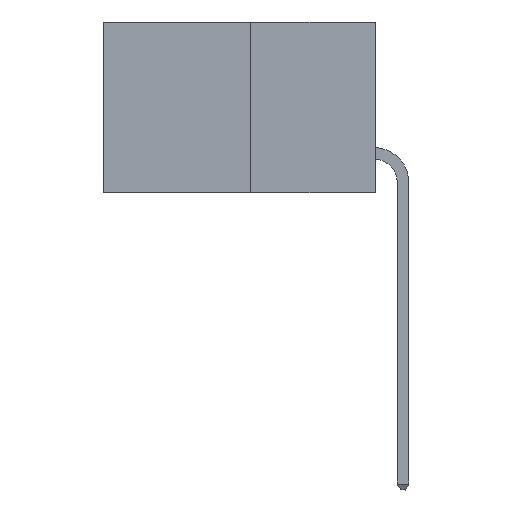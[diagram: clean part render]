
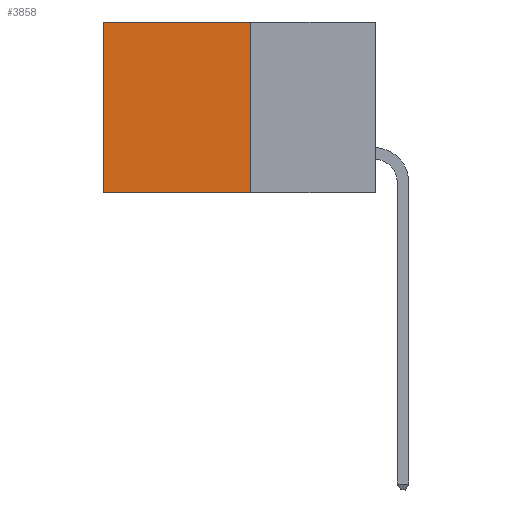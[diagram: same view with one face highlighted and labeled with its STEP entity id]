
A CAD part, left-side view. The second image highlights one B-rep face of the part: STEP entity #3858.
In plain terms, the highlighted planar face has unit normal (-1, 0, 0).
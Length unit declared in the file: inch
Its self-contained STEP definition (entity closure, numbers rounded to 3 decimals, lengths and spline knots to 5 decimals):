
#7 = DIRECTION ( 'NONE',  ( 1., 0., 0. ) ) ;
#21 = CARTESIAN_POINT ( 'NONE',  ( 0.277, 0.59, 0. ) ) ;
#32 = DIRECTION ( 'NONE',  ( 0., 0., -1. ) ) ;
#64 = CARTESIAN_POINT ( 'NONE',  ( 0.277, 0.59, -0.37 ) ) ;
#300 = VECTOR ( 'NONE', #7304, 39.37008 ) ;
#624 = VERTEX_POINT ( 'NONE', #8004 ) ;
#663 = VERTEX_POINT ( 'NONE', #3775 ) ;
#754 = CARTESIAN_POINT ( 'NONE',  ( 0.277, 0.27, -0.37 ) ) ;
#765 = ORIENTED_EDGE ( 'NONE', *, *, #2638, .T. ) ;
#917 = VECTOR ( 'NONE', #32, 39.37008 ) ;
#1384 = ORIENTED_EDGE ( 'NONE', *, *, #1924, .T. ) ;
#1499 = VERTEX_POINT ( 'NONE', #21 ) ;
#1924 = EDGE_CURVE ( 'NONE', #663, #1499, #2099, .T. ) ;
#2035 = DIRECTION ( 'NONE',  ( 0., 1., 0. ) ) ;
#2059 = FACE_OUTER_BOUND ( 'NONE', #2167, .T. ) ;
#2099 = LINE ( 'NONE', #4735, #7469 ) ;
#2167 = EDGE_LOOP ( 'NONE', ( #765, #7737, #5926, #1384 ) ) ;
#2505 = LINE ( 'NONE', #7928, #300 ) ;
#2638 = EDGE_CURVE ( 'NONE', #1499, #6406, #6531, .T. ) ;
#2946 = VECTOR ( 'NONE', #2035, 39.37008 ) ;
#3775 = CARTESIAN_POINT ( 'NONE',  ( 0.277, 0.27, 0. ) ) ;
#3858 = ADVANCED_FACE ( 'NONE', ( #2059 ), #5508, .F. ) ;
#4472 = LINE ( 'NONE', #7286, #2946 ) ;
#4735 = CARTESIAN_POINT ( 'NONE',  ( 0.277, 0.27, 0. ) ) ;
#5428 = DIRECTION ( 'NONE',  ( 0., 0., -1. ) ) ;
#5490 = CARTESIAN_POINT ( 'NONE',  ( 0.277, 0.59, -0.37 ) ) ;
#5508 = PLANE ( 'NONE',  #6463 ) ;
#5926 = ORIENTED_EDGE ( 'NONE', *, *, #7028, .F. ) ;
#6406 = VERTEX_POINT ( 'NONE', #5490 ) ;
#6463 = AXIS2_PLACEMENT_3D ( 'NONE', #754, #7, #5428 ) ;
#6531 = LINE ( 'NONE', #64, #917 ) ;
#7028 = EDGE_CURVE ( 'NONE', #663, #624, #2505, .T. ) ;
#7286 = CARTESIAN_POINT ( 'NONE',  ( 0.277, 0.27, -0.37 ) ) ;
#7304 = DIRECTION ( 'NONE',  ( 0., 0., -1. ) ) ;
#7469 = VECTOR ( 'NONE', #8106, 39.37008 ) ;
#7737 = ORIENTED_EDGE ( 'NONE', *, *, #7942, .F. ) ;
#7928 = CARTESIAN_POINT ( 'NONE',  ( 0.277, 0.27, -0.37 ) ) ;
#7942 = EDGE_CURVE ( 'NONE', #624, #6406, #4472, .T. ) ;
#8004 = CARTESIAN_POINT ( 'NONE',  ( 0.277, 0.27, -0.37 ) ) ;
#8106 = DIRECTION ( 'NONE',  ( 0., 1., 0. ) ) ;
